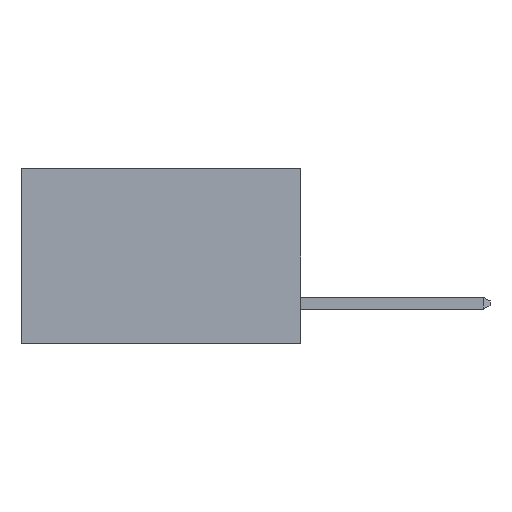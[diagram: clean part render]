
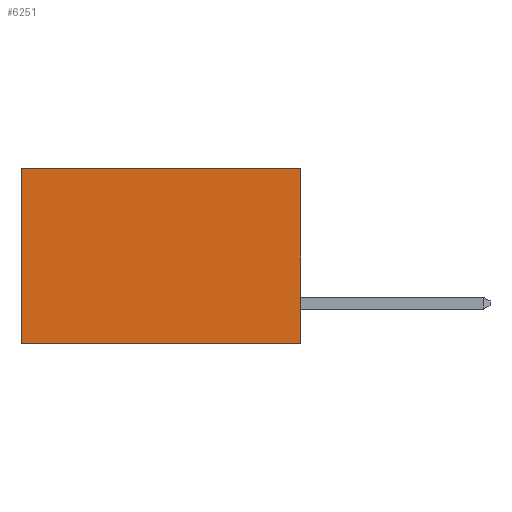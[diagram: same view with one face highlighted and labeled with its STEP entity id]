
A CAD part, left-side view. The second image highlights one B-rep face of the part: STEP entity #6251.
In plain terms, the highlighted planar face has unit normal (-1, 0, 0).
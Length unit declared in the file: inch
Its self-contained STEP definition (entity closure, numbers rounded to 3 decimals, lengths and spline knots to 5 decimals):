
#104 = LINE ( 'NONE', #3814, #6394 ) ;
#288 = LINE ( 'NONE', #4022, #8347 ) ;
#493 = LINE ( 'NONE', #7369, #4419 ) ;
#697 = CARTESIAN_POINT ( 'NONE',  ( 0.277, 0.59, 0. ) ) ;
#1128 = VERTEX_POINT ( 'NONE', #697 ) ;
#1348 = ORIENTED_EDGE ( 'NONE', *, *, #2778, .F. ) ;
#2307 = CARTESIAN_POINT ( 'NONE',  ( 0.277, 0., 0. ) ) ;
#2590 = CARTESIAN_POINT ( 'NONE',  ( 0.277, 0., -0.37 ) ) ;
#2635 = ORIENTED_EDGE ( 'NONE', *, *, #10201, .T. ) ;
#2778 = EDGE_CURVE ( 'NONE', #4860, #8171, #493, .T. ) ;
#2812 = EDGE_LOOP ( 'NONE', ( #2635, #8753, #1348, #5731 ) ) ;
#2950 = VECTOR ( 'NONE', #3273, 39.37008 ) ;
#3194 = CARTESIAN_POINT ( 'NONE',  ( 0.277, 0., 0. ) ) ;
#3273 = DIRECTION ( 'NONE',  ( 0., 1., 0. ) ) ;
#3392 = PLANE ( 'NONE',  #7392 ) ;
#3814 = CARTESIAN_POINT ( 'NONE',  ( 0.277, 0.59, -0.37 ) ) ;
#4022 = CARTESIAN_POINT ( 'NONE',  ( 0.277, 0., -0.37 ) ) ;
#4419 = VECTOR ( 'NONE', #7389, 39.37008 ) ;
#4654 = VERTEX_POINT ( 'NONE', #9028 ) ;
#4860 = VERTEX_POINT ( 'NONE', #2307 ) ;
#5110 = DIRECTION ( 'NONE',  ( 1., 0., 0. ) ) ;
#5125 = DIRECTION ( 'NONE',  ( 0., 0., -1. ) ) ;
#5198 = CARTESIAN_POINT ( 'NONE',  ( 0.277, 0., -0.37 ) ) ;
#5709 = FACE_OUTER_BOUND ( 'NONE', #2812, .T. ) ;
#5731 = ORIENTED_EDGE ( 'NONE', *, *, #6502, .T. ) ;
#5976 = EDGE_CURVE ( 'NONE', #8171, #4654, #288, .T. ) ;
#6251 = ADVANCED_FACE ( 'NONE', ( #5709 ), #3392, .F. ) ;
#6394 = VECTOR ( 'NONE', #7723, 39.37008 ) ;
#6502 = EDGE_CURVE ( 'NONE', #4860, #1128, #7135, .T. ) ;
#7135 = LINE ( 'NONE', #3194, #2950 ) ;
#7227 = DIRECTION ( 'NONE',  ( 0., 1., 0. ) ) ;
#7369 = CARTESIAN_POINT ( 'NONE',  ( 0.277, 0., -0.37 ) ) ;
#7389 = DIRECTION ( 'NONE',  ( 0., 0., -1. ) ) ;
#7392 = AXIS2_PLACEMENT_3D ( 'NONE', #5198, #5110, #5125 ) ;
#7723 = DIRECTION ( 'NONE',  ( 0., 0., -1. ) ) ;
#8171 = VERTEX_POINT ( 'NONE', #2590 ) ;
#8347 = VECTOR ( 'NONE', #7227, 39.37008 ) ;
#8753 = ORIENTED_EDGE ( 'NONE', *, *, #5976, .F. ) ;
#9028 = CARTESIAN_POINT ( 'NONE',  ( 0.277, 0.59, -0.37 ) ) ;
#10201 = EDGE_CURVE ( 'NONE', #1128, #4654, #104, .T. ) ;
